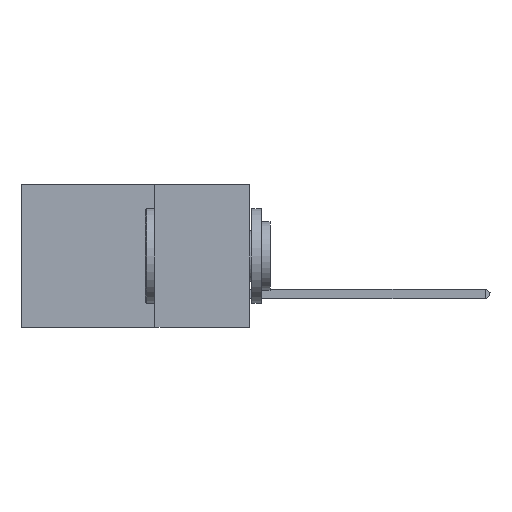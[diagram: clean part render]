
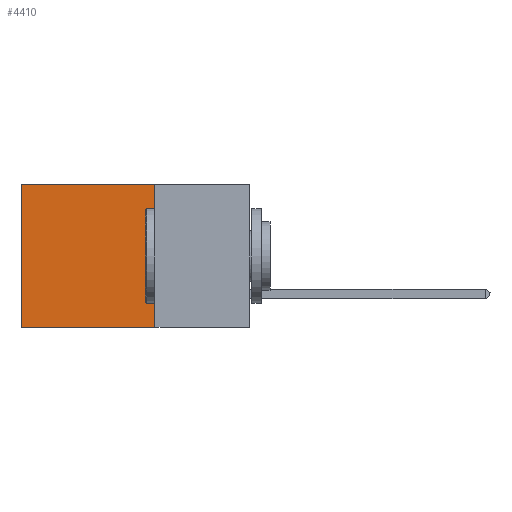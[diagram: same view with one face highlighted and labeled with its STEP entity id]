
A CAD part, left-side view. The second image highlights one B-rep face of the part: STEP entity #4410.
In plain terms, the highlighted planar face has unit normal (-1, 0, 0).
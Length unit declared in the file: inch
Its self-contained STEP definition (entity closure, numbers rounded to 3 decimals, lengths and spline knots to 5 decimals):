
#87 = VECTOR ( 'NONE', #8208, 39.37008 ) ;
#424 = ORIENTED_EDGE ( 'NONE', *, *, #2927, .F. ) ;
#1770 = LINE ( 'NONE', #9330, #87 ) ;
#1851 = CARTESIAN_POINT ( 'NONE',  ( 0.2875, 0.25, -0.375 ) ) ;
#2426 = VECTOR ( 'NONE', #13176, 39.37008 ) ;
#2826 = DIRECTION ( 'NONE',  ( 0., 0., -1. ) ) ;
#2927 = EDGE_CURVE ( 'NONE', #5388, #6641, #1770, .T. ) ;
#3802 = CARTESIAN_POINT ( 'NONE',  ( 0.2875, 0.6, -0.375 ) ) ;
#4410 = ADVANCED_FACE ( 'NONE', ( #7192 ), #9303, .F. ) ;
#5388 = VERTEX_POINT ( 'NONE', #1851 ) ;
#5486 = CARTESIAN_POINT ( 'NONE',  ( 0.2875, 0.6, 0. ) ) ;
#5600 = CARTESIAN_POINT ( 'NONE',  ( 0.2875, 0.6, -0.375 ) ) ;
#6365 = CARTESIAN_POINT ( 'NONE',  ( 0.2875, 0.25, 0. ) ) ;
#6641 = VERTEX_POINT ( 'NONE', #3802 ) ;
#7192 = FACE_OUTER_BOUND ( 'NONE', #7917, .T. ) ;
#7284 = DIRECTION ( 'NONE',  ( 0., 1., 0. ) ) ;
#7416 = LINE ( 'NONE', #6365, #9152 ) ;
#7917 = EDGE_LOOP ( 'NONE', ( #8789, #424, #11707, #9677 ) ) ;
#8127 = VERTEX_POINT ( 'NONE', #12848 ) ;
#8179 = DIRECTION ( 'NONE',  ( 0., 0., -1. ) ) ;
#8208 = DIRECTION ( 'NONE',  ( 0., 1., 0. ) ) ;
#8319 = DIRECTION ( 'NONE',  ( 1., 0., 0. ) ) ;
#8775 = LINE ( 'NONE', #5600, #2426 ) ;
#8789 = ORIENTED_EDGE ( 'NONE', *, *, #13509, .T. ) ;
#9143 = VECTOR ( 'NONE', #2826, 39.37008 ) ;
#9152 = VECTOR ( 'NONE', #7284, 39.37008 ) ;
#9303 = PLANE ( 'NONE',  #13679 ) ;
#9330 = CARTESIAN_POINT ( 'NONE',  ( 0.2875, 0.25, -0.375 ) ) ;
#9677 = ORIENTED_EDGE ( 'NONE', *, *, #13766, .T. ) ;
#9805 = VERTEX_POINT ( 'NONE', #5486 ) ;
#11452 = LINE ( 'NONE', #13674, #9143 ) ;
#11707 = ORIENTED_EDGE ( 'NONE', *, *, #13157, .F. ) ;
#12848 = CARTESIAN_POINT ( 'NONE',  ( 0.2875, 0.25, 0. ) ) ;
#13157 = EDGE_CURVE ( 'NONE', #8127, #5388, #11452, .T. ) ;
#13176 = DIRECTION ( 'NONE',  ( 0., 0., -1. ) ) ;
#13509 = EDGE_CURVE ( 'NONE', #9805, #6641, #8775, .T. ) ;
#13568 = CARTESIAN_POINT ( 'NONE',  ( 0.2875, 0.25, -0.375 ) ) ;
#13674 = CARTESIAN_POINT ( 'NONE',  ( 0.2875, 0.25, -0.375 ) ) ;
#13679 = AXIS2_PLACEMENT_3D ( 'NONE', #13568, #8319, #8179 ) ;
#13766 = EDGE_CURVE ( 'NONE', #8127, #9805, #7416, .T. ) ;
